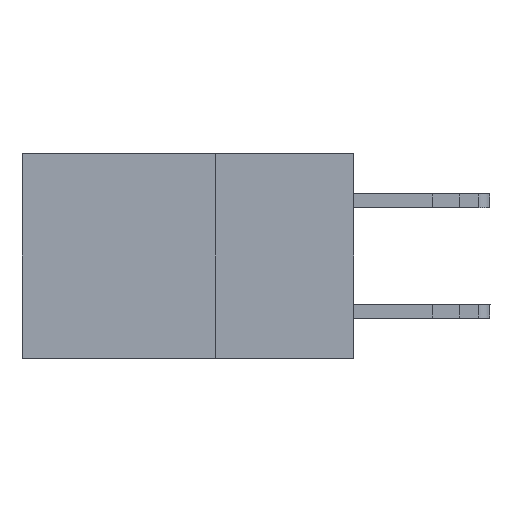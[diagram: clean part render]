
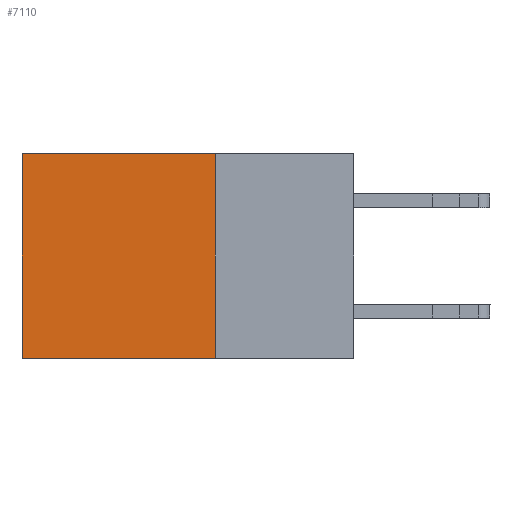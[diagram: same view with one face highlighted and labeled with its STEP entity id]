
A CAD part, left-side view. The second image highlights one B-rep face of the part: STEP entity #7110.
In plain terms, the highlighted planar face has unit normal (-1, 0, 0).
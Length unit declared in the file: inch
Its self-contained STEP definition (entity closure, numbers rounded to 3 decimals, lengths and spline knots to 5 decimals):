
#129 = EDGE_CURVE ( 'NONE', #604, #26976, #5704, .T. ) ;
#199 = DIRECTION ( 'NONE',  ( 1., 0., 0. ) ) ;
#312 = VECTOR ( 'NONE', #21006, 39.37008 ) ;
#320 = CARTESIAN_POINT ( 'NONE',  ( 0.2875, 0.25, 0. ) ) ;
#604 = VERTEX_POINT ( 'NONE', #7718 ) ;
#2009 = AXIS2_PLACEMENT_3D ( 'NONE', #10749, #199, #14720 ) ;
#2353 = LINE ( 'NONE', #320, #312 ) ;
#2801 = VECTOR ( 'NONE', #14509, 39.37008 ) ;
#3113 = CARTESIAN_POINT ( 'NONE',  ( 0.2875, 0.25, -0.37 ) ) ;
#5704 = LINE ( 'NONE', #10228, #6687 ) ;
#6687 = VECTOR ( 'NONE', #10513, 39.37008 ) ;
#7110 = ADVANCED_FACE ( 'NONE', ( #25256 ), #23200, .F. ) ;
#7718 = CARTESIAN_POINT ( 'NONE',  ( 0.2875, 0.25, 0. ) ) ;
#8253 = CARTESIAN_POINT ( 'NONE',  ( 0.2875, 0.6, -0.37 ) ) ;
#9020 = LINE ( 'NONE', #3113, #9454 ) ;
#9284 = EDGE_CURVE ( 'NONE', #604, #12271, #2353, .T. ) ;
#9454 = VECTOR ( 'NONE', #23940, 39.37008 ) ;
#9490 = ORIENTED_EDGE ( 'NONE', *, *, #129, .T. ) ;
#10228 = CARTESIAN_POINT ( 'NONE',  ( 0.2875, 0.25, 0. ) ) ;
#10513 = DIRECTION ( 'NONE',  ( 0., 1., 0. ) ) ;
#10543 = LINE ( 'NONE', #12453, #2801 ) ;
#10749 = CARTESIAN_POINT ( 'NONE',  ( 0.2875, 0.25, 0. ) ) ;
#10969 = EDGE_LOOP ( 'NONE', ( #23747, #16115, #16638, #9490 ) ) ;
#12271 = VERTEX_POINT ( 'NONE', #17712 ) ;
#12453 = CARTESIAN_POINT ( 'NONE',  ( 0.2875, 0.6, 0. ) ) ;
#13142 = EDGE_CURVE ( 'NONE', #12271, #23759, #9020, .T. ) ;
#14509 = DIRECTION ( 'NONE',  ( 0., 0., -1. ) ) ;
#14720 = DIRECTION ( 'NONE',  ( 0., 0., -1. ) ) ;
#16115 = ORIENTED_EDGE ( 'NONE', *, *, #13142, .F. ) ;
#16638 = ORIENTED_EDGE ( 'NONE', *, *, #9284, .F. ) ;
#17712 = CARTESIAN_POINT ( 'NONE',  ( 0.2875, 0.25, -0.37 ) ) ;
#18924 = CARTESIAN_POINT ( 'NONE',  ( 0.2875, 0.6, 0. ) ) ;
#21006 = DIRECTION ( 'NONE',  ( 0., 0., -1. ) ) ;
#21766 = EDGE_CURVE ( 'NONE', #26976, #23759, #10543, .T. ) ;
#23200 = PLANE ( 'NONE',  #2009 ) ;
#23747 = ORIENTED_EDGE ( 'NONE', *, *, #21766, .T. ) ;
#23759 = VERTEX_POINT ( 'NONE', #8253 ) ;
#23940 = DIRECTION ( 'NONE',  ( 0., 1., 0. ) ) ;
#25256 = FACE_OUTER_BOUND ( 'NONE', #10969, .T. ) ;
#26976 = VERTEX_POINT ( 'NONE', #18924 ) ;
